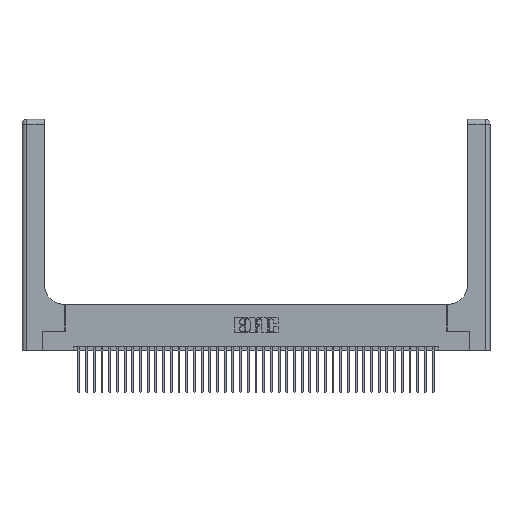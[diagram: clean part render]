
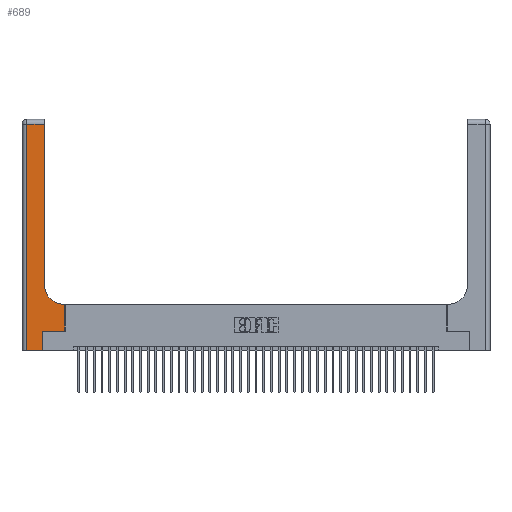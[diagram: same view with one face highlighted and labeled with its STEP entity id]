
A CAD part, top view. The second image highlights one B-rep face of the part: STEP entity #689.
In plain terms, the highlighted planar face has unit normal (0, 0, 1).
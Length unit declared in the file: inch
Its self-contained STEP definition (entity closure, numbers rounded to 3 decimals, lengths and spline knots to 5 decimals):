
#105 = VECTOR ( 'NONE', #19072, 39.37008 ) ;
#231 = CARTESIAN_POINT ( 'NONE',  ( 0.2915, 2.94, 0.37 ) ) ;
#454 = LINE ( 'NONE', #11815, #16478 ) ;
#670 = DIRECTION ( 'NONE',  ( 1., 0., 0. ) ) ;
#689 = ADVANCED_FACE ( 'NONE', ( #26049 ), #24622, .F. ) ;
#784 = VECTOR ( 'NONE', #1930, 39.37008 ) ;
#843 = EDGE_CURVE ( 'NONE', #14047, #34637, #3041, .T. ) ;
#1405 = CARTESIAN_POINT ( 'NONE',  ( 0.5585, 0.25, 0.37 ) ) ;
#1930 = DIRECTION ( 'NONE',  ( 0., -1., 0. ) ) ;
#2006 = LINE ( 'NONE', #16161, #26498 ) ;
#2161 = ORIENTED_EDGE ( 'NONE', *, *, #37424, .T. ) ;
#3041 = LINE ( 'NONE', #25847, #4068 ) ;
#3197 = CARTESIAN_POINT ( 'NONE',  ( 0.269, 0., 0.37 ) ) ;
#3281 = CARTESIAN_POINT ( 'NONE',  ( 0.06, 2.94, 0.37 ) ) ;
#3617 = LINE ( 'NONE', #9767, #20627 ) ;
#4068 = VECTOR ( 'NONE', #9935, 39.37008 ) ;
#6363 = ORIENTED_EDGE ( 'NONE', *, *, #40993, .T. ) ;
#6674 = EDGE_CURVE ( 'NONE', #9229, #22630, #17801, .T. ) ;
#9229 = VERTEX_POINT ( 'NONE', #3281 ) ;
#9767 = CARTESIAN_POINT ( 'NONE',  ( 0., 0., 0.37 ) ) ;
#9935 = DIRECTION ( 'NONE',  ( 1., 0., 0. ) ) ;
#10249 = ORIENTED_EDGE ( 'NONE', *, *, #40930, .T. ) ;
#10678 = CARTESIAN_POINT ( 'NONE',  ( 0.06, 0., 0.37 ) ) ;
#11130 = ORIENTED_EDGE ( 'NONE', *, *, #40394, .T. ) ;
#11815 = CARTESIAN_POINT ( 'NONE',  ( 0.5585, 0.25, 0.37 ) ) ;
#12689 = EDGE_CURVE ( 'NONE', #21783, #14047, #23639, .T. ) ;
#13667 = EDGE_LOOP ( 'NONE', ( #6363, #10249, #29414, #40603, #34271, #32690, #24098, #11130, #2161 ) ) ;
#14047 = VERTEX_POINT ( 'NONE', #35189 ) ;
#14420 = VERTEX_POINT ( 'NONE', #231 ) ;
#15090 = DIRECTION ( 'NONE',  ( -1., 0., 0. ) ) ;
#15776 = CARTESIAN_POINT ( 'NONE',  ( 0., 2.94, 0.37 ) ) ;
#16161 = CARTESIAN_POINT ( 'NONE',  ( 0.2915, 3., 0.37 ) ) ;
#16478 = VECTOR ( 'NONE', #24547, 39.37008 ) ;
#16536 = DIRECTION ( 'NONE',  ( -1., 0., 0. ) ) ;
#17569 = LINE ( 'NONE', #38901, #41043 ) ;
#17801 = LINE ( 'NONE', #40343, #784 ) ;
#18267 = AXIS2_PLACEMENT_3D ( 'NONE', #27815, #34275, #15090 ) ;
#19072 = DIRECTION ( 'NONE',  ( 0., 1., 0. ) ) ;
#19844 = DIRECTION ( 'NONE',  ( 0., 0., -1. ) ) ;
#20627 = VECTOR ( 'NONE', #32112, 39.37008 ) ;
#21783 = VERTEX_POINT ( 'NONE', #3197 ) ;
#22008 = LINE ( 'NONE', #15776, #39013 ) ;
#22630 = VERTEX_POINT ( 'NONE', #10678 ) ;
#23639 = LINE ( 'NONE', #38195, #105 ) ;
#24098 = ORIENTED_EDGE ( 'NONE', *, *, #41299, .T. ) ;
#24547 = DIRECTION ( 'NONE',  ( 0., 1., 0. ) ) ;
#24622 = PLANE ( 'NONE',  #18267 ) ;
#25847 = CARTESIAN_POINT ( 'NONE',  ( 0.269, 0.25, 0.37 ) ) ;
#26049 = FACE_OUTER_BOUND ( 'NONE', #13667, .T. ) ;
#26498 = VECTOR ( 'NONE', #35316, 39.37008 ) ;
#27297 = AXIS2_PLACEMENT_3D ( 'NONE', #38968, #19844, #670 ) ;
#27467 = EDGE_CURVE ( 'NONE', #22630, #21783, #3617, .T. ) ;
#27815 = CARTESIAN_POINT ( 'NONE',  ( 0., 3., 0.37 ) ) ;
#27963 = CARTESIAN_POINT ( 'NONE',  ( 0.5415, 0.6, 0.37 ) ) ;
#29414 = ORIENTED_EDGE ( 'NONE', *, *, #6674, .T. ) ;
#31375 = CARTESIAN_POINT ( 'NONE',  ( 0.5585, 0.6, 0.37 ) ) ;
#31743 = CIRCLE ( 'NONE', #27297, 0.25 ) ;
#31745 = VERTEX_POINT ( 'NONE', #31375 ) ;
#32112 = DIRECTION ( 'NONE',  ( 1., 0., 0. ) ) ;
#32690 = ORIENTED_EDGE ( 'NONE', *, *, #843, .T. ) ;
#33587 = VERTEX_POINT ( 'NONE', #34747 ) ;
#34271 = ORIENTED_EDGE ( 'NONE', *, *, #12689, .T. ) ;
#34275 = DIRECTION ( 'NONE',  ( 0., 0., -1. ) ) ;
#34637 = VERTEX_POINT ( 'NONE', #1405 ) ;
#34747 = CARTESIAN_POINT ( 'NONE',  ( 0.2915, 0.85, 0.37 ) ) ;
#34944 = DIRECTION ( 'NONE',  ( -1., 0., 0. ) ) ;
#35189 = CARTESIAN_POINT ( 'NONE',  ( 0.269, 0.25, 0.37 ) ) ;
#35316 = DIRECTION ( 'NONE',  ( 0., 1., 0. ) ) ;
#36545 = VERTEX_POINT ( 'NONE', #27963 ) ;
#37424 = EDGE_CURVE ( 'NONE', #36545, #33587, #31743, .T. ) ;
#38195 = CARTESIAN_POINT ( 'NONE',  ( 0.269, 0., 0.37 ) ) ;
#38901 = CARTESIAN_POINT ( 'NONE',  ( 0.2915, 0.6, 0.37 ) ) ;
#38968 = CARTESIAN_POINT ( 'NONE',  ( 0.5415, 0.85, 0.37 ) ) ;
#39013 = VECTOR ( 'NONE', #34944, 39.37008 ) ;
#40343 = CARTESIAN_POINT ( 'NONE',  ( 0.06, 3., 0.37 ) ) ;
#40394 = EDGE_CURVE ( 'NONE', #31745, #36545, #17569, .T. ) ;
#40603 = ORIENTED_EDGE ( 'NONE', *, *, #27467, .T. ) ;
#40930 = EDGE_CURVE ( 'NONE', #14420, #9229, #22008, .T. ) ;
#40993 = EDGE_CURVE ( 'NONE', #33587, #14420, #2006, .T. ) ;
#41043 = VECTOR ( 'NONE', #16536, 39.37008 ) ;
#41299 = EDGE_CURVE ( 'NONE', #34637, #31745, #454, .T. ) ;
